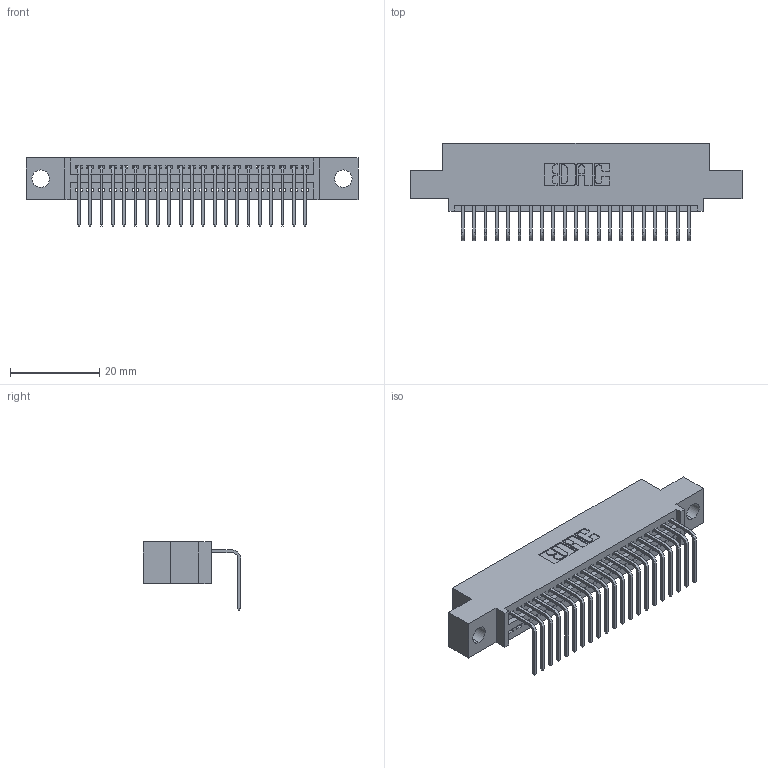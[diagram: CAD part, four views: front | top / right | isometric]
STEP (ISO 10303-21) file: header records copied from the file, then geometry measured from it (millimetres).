
FILE_DESCRIPTION (( 'STEP AP203' ), '1' );
FILE_NAME ('395-021-558-404.STEP', '2021-06-11T14:16:04', ( '' ), ( '' ), 'SwSTEP 2.0', 'SolidWorks 2020', '' );
FILE_SCHEMA (( 'CONFIG_CONTROL_DESIGN' ));
Length unit declared in the file: inch
Products named in the file (3): 395-021-558-404; 345 Part_0.110 Offset - 0.156 Dia-TI; 345-292-001_558 Tail - 2
Assembly tree (22 placements, depth 2):
  395-021-558-404
    345 Part_0.110 Offset - 0.156 Dia-TI
    345-292-001_558 Tail - 2  x21
Bounding box: 74.55 x 21.83 x 15.37 mm (x, y, z)
Volume: 6799.4 mm3; surface area: 9085.8 mm2
Topology: 22 solids, 22 shells, 1404 faces, 4211 edges, 2778 vertices
Faces by surface type: plane 980, cylinder 424
Entity records: 19267 total; most frequent: CARTESIAN_POINT 3349, ORIENTED_EDGE 3302, DIRECTION 2953, EDGE_CURVE 1651, VECTOR 1435, LINE 1435, VERTEX_POINT 1098, AXIS2_PLACEMENT_3D 759
